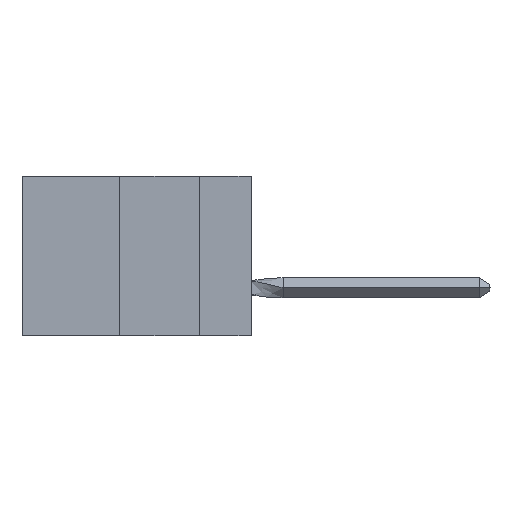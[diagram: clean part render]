
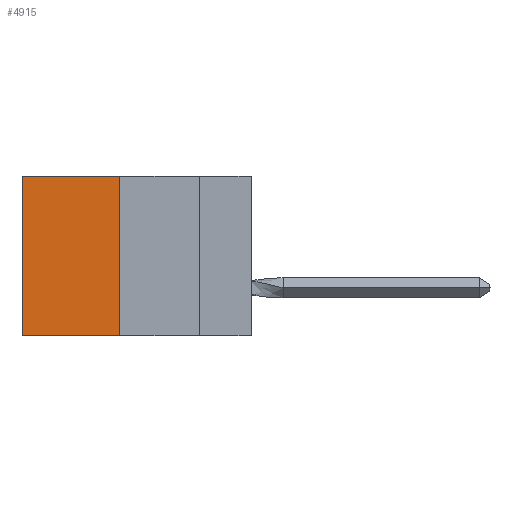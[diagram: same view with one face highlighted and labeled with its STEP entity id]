
A CAD part, left-side view. The second image highlights one B-rep face of the part: STEP entity #4915.
In plain terms, the highlighted planar face has unit normal (-1, 0, 0).
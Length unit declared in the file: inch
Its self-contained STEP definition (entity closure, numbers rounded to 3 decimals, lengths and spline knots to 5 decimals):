
#287 = AXIS2_PLACEMENT_3D ( 'NONE', #13489, #3943, #9607 ) ;
#784 = CARTESIAN_POINT ( 'NONE',  ( 0.305, 0.72, -0.5 ) ) ;
#995 = ORIENTED_EDGE ( 'NONE', *, *, #12921, .F. ) ;
#1220 = CARTESIAN_POINT ( 'NONE',  ( 0.305, 0.413, -0.5 ) ) ;
#1611 = LINE ( 'NONE', #2565, #19175 ) ;
#1693 = LINE ( 'NONE', #5059, #20217 ) ;
#2264 = VERTEX_POINT ( 'NONE', #784 ) ;
#2565 = CARTESIAN_POINT ( 'NONE',  ( 0.305, 0.72, -0.5 ) ) ;
#3943 = DIRECTION ( 'NONE',  ( 1., 0., 0. ) ) ;
#4102 = EDGE_CURVE ( 'NONE', #14536, #2264, #1611, .T. ) ;
#4915 = ADVANCED_FACE ( 'NONE', ( #13965 ), #9454, .F. ) ;
#5059 = CARTESIAN_POINT ( 'NONE',  ( 0.305, 0.413, -0.5 ) ) ;
#5543 = CARTESIAN_POINT ( 'NONE',  ( 0.305, 0.413, 0. ) ) ;
#6363 = ORIENTED_EDGE ( 'NONE', *, *, #14752, .T. ) ;
#6550 = DIRECTION ( 'NONE',  ( 0., 0., -1. ) ) ;
#8253 = VECTOR ( 'NONE', #10916, 39.37008 ) ;
#9454 = PLANE ( 'NONE',  #287 ) ;
#9607 = DIRECTION ( 'NONE',  ( 0., 0., -1. ) ) ;
#10658 = LINE ( 'NONE', #5543, #8253 ) ;
#10891 = ORIENTED_EDGE ( 'NONE', *, *, #4102, .T. ) ;
#10916 = DIRECTION ( 'NONE',  ( 0., 1., 0. ) ) ;
#10968 = DIRECTION ( 'NONE',  ( 0., 0., -1. ) ) ;
#12915 = VERTEX_POINT ( 'NONE', #1220 ) ;
#12921 = EDGE_CURVE ( 'NONE', #14845, #12915, #1693, .T. ) ;
#13165 = ORIENTED_EDGE ( 'NONE', *, *, #14183, .F. ) ;
#13375 = CARTESIAN_POINT ( 'NONE',  ( 0.305, 0.413, 0. ) ) ;
#13489 = CARTESIAN_POINT ( 'NONE',  ( 0.305, 0.413, -0.5 ) ) ;
#13812 = CARTESIAN_POINT ( 'NONE',  ( 0.305, 0.72, 0. ) ) ;
#13965 = FACE_OUTER_BOUND ( 'NONE', #19147, .T. ) ;
#14183 = EDGE_CURVE ( 'NONE', #12915, #2264, #16443, .T. ) ;
#14536 = VERTEX_POINT ( 'NONE', #13812 ) ;
#14752 = EDGE_CURVE ( 'NONE', #14845, #14536, #10658, .T. ) ;
#14845 = VERTEX_POINT ( 'NONE', #13375 ) ;
#15825 = VECTOR ( 'NONE', #17858, 39.37008 ) ;
#16443 = LINE ( 'NONE', #23729, #15825 ) ;
#17858 = DIRECTION ( 'NONE',  ( 0., 1., 0. ) ) ;
#19147 = EDGE_LOOP ( 'NONE', ( #10891, #13165, #995, #6363 ) ) ;
#19175 = VECTOR ( 'NONE', #6550, 39.37008 ) ;
#20217 = VECTOR ( 'NONE', #10968, 39.37008 ) ;
#23729 = CARTESIAN_POINT ( 'NONE',  ( 0.305, 0.413, -0.5 ) ) ;
